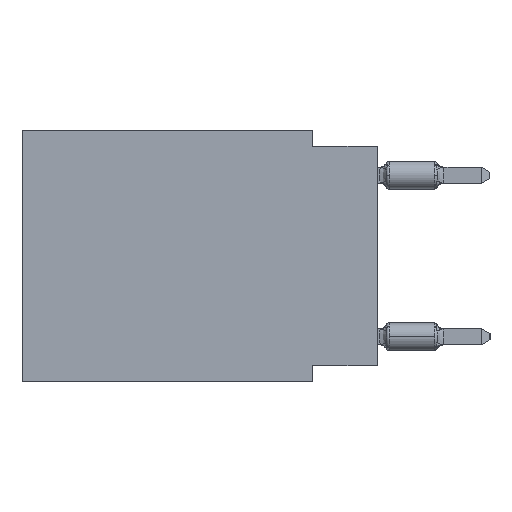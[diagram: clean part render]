
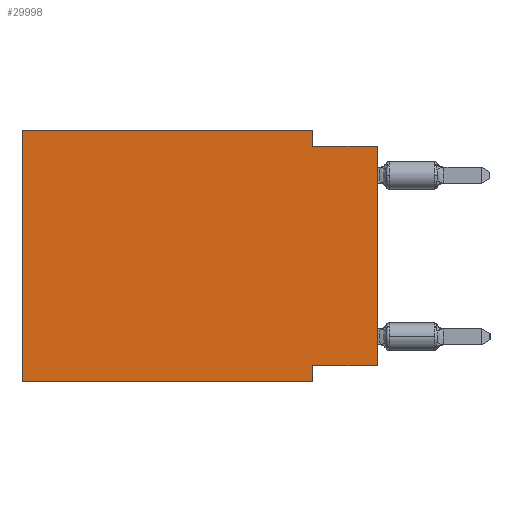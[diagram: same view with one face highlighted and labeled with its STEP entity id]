
A CAD part, left-side view. The second image highlights one B-rep face of the part: STEP entity #29998.
In plain terms, the highlighted planar face has unit normal (-1, 0, 0).
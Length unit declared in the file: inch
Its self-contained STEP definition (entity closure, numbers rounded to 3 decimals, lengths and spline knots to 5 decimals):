
#166 = DIRECTION ( 'NONE',  ( 0., -1., 0. ) ) ;
#338 = ORIENTED_EDGE ( 'NONE', *, *, #23301, .F. ) ;
#676 = VERTEX_POINT ( 'NONE', #28823 ) ;
#730 = EDGE_CURVE ( 'NONE', #25308, #5874, #16526, .T. ) ;
#1078 = CARTESIAN_POINT ( 'NONE',  ( 0., 0., -0.025 ) ) ;
#1079 = DIRECTION ( 'NONE',  ( 0., 0., -1. ) ) ;
#1227 = VERTEX_POINT ( 'NONE', #19729 ) ;
#1464 = VECTOR ( 'NONE', #25280, 39.37008 ) ;
#3135 = FACE_OUTER_BOUND ( 'NONE', #23966, .T. ) ;
#4393 = LINE ( 'NONE', #11473, #16525 ) ;
#5007 = CARTESIAN_POINT ( 'NONE',  ( 0., 0.55, 0. ) ) ;
#5346 = DIRECTION ( 'NONE',  ( 0., 1., 0. ) ) ;
#5874 = VERTEX_POINT ( 'NONE', #12996 ) ;
#6066 = CARTESIAN_POINT ( 'NONE',  ( 0., 0., 0. ) ) ;
#6849 = VECTOR ( 'NONE', #166, 39.37008 ) ;
#7279 = LINE ( 'NONE', #16890, #6849 ) ;
#7953 = VERTEX_POINT ( 'NONE', #22074 ) ;
#8129 = VECTOR ( 'NONE', #14628, 39.37008 ) ;
#8176 = CARTESIAN_POINT ( 'NONE',  ( 0., 0., -0.365 ) ) ;
#8530 = VERTEX_POINT ( 'NONE', #17783 ) ;
#9118 = VERTEX_POINT ( 'NONE', #24136 ) ;
#9659 = EDGE_CURVE ( 'NONE', #7953, #1227, #12443, .T. ) ;
#9912 = EDGE_CURVE ( 'NONE', #9118, #8530, #21244, .T. ) ;
#11009 = VECTOR ( 'NONE', #28280, 39.37008 ) ;
#11473 = CARTESIAN_POINT ( 'NONE',  ( 0., 0.1, -0.39 ) ) ;
#11912 = ORIENTED_EDGE ( 'NONE', *, *, #24174, .T. ) ;
#12443 = LINE ( 'NONE', #8176, #17196 ) ;
#12753 = LINE ( 'NONE', #1078, #25144 ) ;
#12996 = CARTESIAN_POINT ( 'NONE',  ( 0., 0.1, -0.025 ) ) ;
#13033 = ORIENTED_EDGE ( 'NONE', *, *, #9659, .F. ) ;
#13428 = VERTEX_POINT ( 'NONE', #19450 ) ;
#13950 = VECTOR ( 'NONE', #16215, 39.37008 ) ;
#14553 = EDGE_CURVE ( 'NONE', #7953, #13428, #27659, .T. ) ;
#14628 = DIRECTION ( 'NONE',  ( 0., 0., 1. ) ) ;
#15068 = ORIENTED_EDGE ( 'NONE', *, *, #9912, .F. ) ;
#15571 = ORIENTED_EDGE ( 'NONE', *, *, #14553, .T. ) ;
#16215 = DIRECTION ( 'NONE',  ( 0., 0., -1. ) ) ;
#16525 = VECTOR ( 'NONE', #28826, 39.37008 ) ;
#16526 = LINE ( 'NONE', #21090, #13950 ) ;
#16890 = CARTESIAN_POINT ( 'NONE',  ( 0., 0.55, 0. ) ) ;
#17196 = VECTOR ( 'NONE', #5346, 39.37008 ) ;
#17648 = DIRECTION ( 'NONE',  ( 0., -1., 0. ) ) ;
#17783 = CARTESIAN_POINT ( 'NONE',  ( 0., 0.55, 0. ) ) ;
#17913 = ORIENTED_EDGE ( 'NONE', *, *, #730, .F. ) ;
#19130 = LINE ( 'NONE', #21018, #11009 ) ;
#19450 = CARTESIAN_POINT ( 'NONE',  ( 0., 0., -0.025 ) ) ;
#19729 = CARTESIAN_POINT ( 'NONE',  ( 0., 0.1, -0.365 ) ) ;
#19841 = CARTESIAN_POINT ( 'NONE',  ( 0., 0.55, 0. ) ) ;
#20502 = EDGE_CURVE ( 'NONE', #8530, #25308, #7279, .T. ) ;
#21018 = CARTESIAN_POINT ( 'NONE',  ( 0., 0.55, -0.39 ) ) ;
#21090 = CARTESIAN_POINT ( 'NONE',  ( 0., 0.1, 0. ) ) ;
#21244 = LINE ( 'NONE', #5007, #8129 ) ;
#22074 = CARTESIAN_POINT ( 'NONE',  ( 0., 0., -0.365 ) ) ;
#22506 = ORIENTED_EDGE ( 'NONE', *, *, #24883, .F. ) ;
#22556 = ORIENTED_EDGE ( 'NONE', *, *, #20502, .F. ) ;
#23301 = EDGE_CURVE ( 'NONE', #1227, #676, #4393, .T. ) ;
#23966 = EDGE_LOOP ( 'NONE', ( #15571, #22506, #17913, #22556, #15068, #11912, #338, #13033 ) ) ;
#24136 = CARTESIAN_POINT ( 'NONE',  ( 0., 0.55, -0.39 ) ) ;
#24174 = EDGE_CURVE ( 'NONE', #9118, #676, #19130, .T. ) ;
#24568 = DIRECTION ( 'NONE',  ( 1., 0., 0. ) ) ;
#24883 = EDGE_CURVE ( 'NONE', #5874, #13428, #12753, .T. ) ;
#25144 = VECTOR ( 'NONE', #17648, 39.37008 ) ;
#25280 = DIRECTION ( 'NONE',  ( 0., 0., 1. ) ) ;
#25308 = VERTEX_POINT ( 'NONE', #27497 ) ;
#26945 = PLANE ( 'NONE',  #29475 ) ;
#27497 = CARTESIAN_POINT ( 'NONE',  ( 0., 0.1, 0. ) ) ;
#27659 = LINE ( 'NONE', #6066, #1464 ) ;
#28280 = DIRECTION ( 'NONE',  ( 0., -1., 0. ) ) ;
#28823 = CARTESIAN_POINT ( 'NONE',  ( 0., 0.1, -0.39 ) ) ;
#28826 = DIRECTION ( 'NONE',  ( 0., 0., -1. ) ) ;
#29475 = AXIS2_PLACEMENT_3D ( 'NONE', #19841, #24568, #1079 ) ;
#29998 = ADVANCED_FACE ( 'NONE', ( #3135 ), #26945, .F. ) ;
